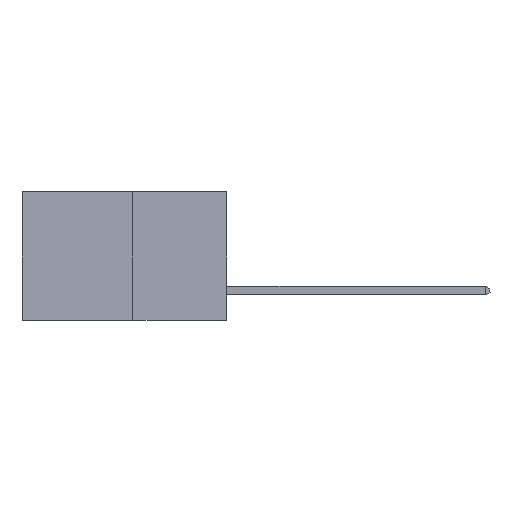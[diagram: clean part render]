
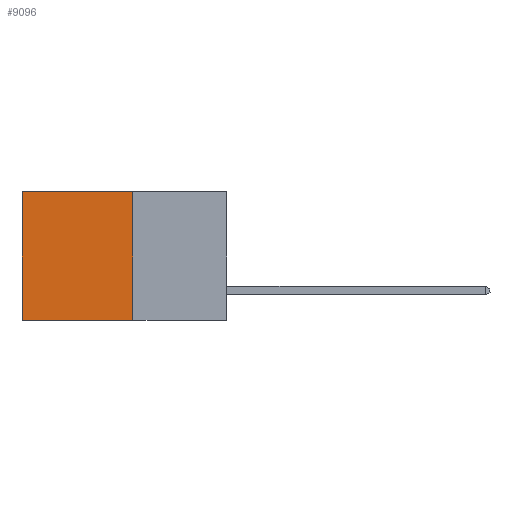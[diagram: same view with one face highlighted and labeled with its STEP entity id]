
A CAD part, left-side view. The second image highlights one B-rep face of the part: STEP entity #9096.
In plain terms, the highlighted planar face has unit normal (-1, 0, 0).
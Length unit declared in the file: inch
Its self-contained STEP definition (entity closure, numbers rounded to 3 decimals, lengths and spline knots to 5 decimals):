
#152 = LINE ( 'NONE', #2036, #10511 ) ;
#272 = VERTEX_POINT ( 'NONE', #1873 ) ;
#310 = VECTOR ( 'NONE', #3339, 39.37008 ) ;
#733 = CARTESIAN_POINT ( 'NONE',  ( 0.277, 0.27, 0. ) ) ;
#773 = ORIENTED_EDGE ( 'NONE', *, *, #8752, .F. ) ;
#1008 = DIRECTION ( 'NONE',  ( 0., 0., -1. ) ) ;
#1807 = DIRECTION ( 'NONE',  ( 1., 0., 0. ) ) ;
#1873 = CARTESIAN_POINT ( 'NONE',  ( 0.277, 0.27, -0.37 ) ) ;
#2036 = CARTESIAN_POINT ( 'NONE',  ( 0.277, 0.27, -0.37 ) ) ;
#2750 = VERTEX_POINT ( 'NONE', #10071 ) ;
#3150 = CARTESIAN_POINT ( 'NONE',  ( 0.277, 0.27, -0.37 ) ) ;
#3339 = DIRECTION ( 'NONE',  ( 0., 1., 0. ) ) ;
#3809 = ORIENTED_EDGE ( 'NONE', *, *, #11280, .T. ) ;
#3997 = CARTESIAN_POINT ( 'NONE',  ( 0.277, 0.59, -0.37 ) ) ;
#4216 = VERTEX_POINT ( 'NONE', #6835 ) ;
#4454 = EDGE_LOOP ( 'NONE', ( #8156, #773, #6133, #3809 ) ) ;
#4616 = VECTOR ( 'NONE', #10073, 39.37008 ) ;
#4999 = DIRECTION ( 'NONE',  ( 0., 0., -1. ) ) ;
#6133 = ORIENTED_EDGE ( 'NONE', *, *, #7423, .F. ) ;
#6651 = VECTOR ( 'NONE', #4999, 39.37008 ) ;
#6835 = CARTESIAN_POINT ( 'NONE',  ( 0.277, 0.59, 0. ) ) ;
#7266 = LINE ( 'NONE', #3150, #4616 ) ;
#7423 = EDGE_CURVE ( 'NONE', #9100, #272, #152, .T. ) ;
#7792 = CARTESIAN_POINT ( 'NONE',  ( 0.277, 0.27, -0.37 ) ) ;
#7883 = FACE_OUTER_BOUND ( 'NONE', #4454, .T. ) ;
#8156 = ORIENTED_EDGE ( 'NONE', *, *, #11171, .T. ) ;
#8288 = CARTESIAN_POINT ( 'NONE',  ( 0.277, 0.27, 0. ) ) ;
#8657 = LINE ( 'NONE', #8288, #310 ) ;
#8746 = DIRECTION ( 'NONE',  ( 0., 0., -1. ) ) ;
#8752 = EDGE_CURVE ( 'NONE', #272, #2750, #7266, .T. ) ;
#9096 = ADVANCED_FACE ( 'NONE', ( #7883 ), #12636, .F. ) ;
#9100 = VERTEX_POINT ( 'NONE', #733 ) ;
#10071 = CARTESIAN_POINT ( 'NONE',  ( 0.277, 0.59, -0.37 ) ) ;
#10073 = DIRECTION ( 'NONE',  ( 0., 1., 0. ) ) ;
#10264 = AXIS2_PLACEMENT_3D ( 'NONE', #7792, #1807, #8746 ) ;
#10511 = VECTOR ( 'NONE', #1008, 39.37008 ) ;
#11171 = EDGE_CURVE ( 'NONE', #4216, #2750, #12170, .T. ) ;
#11280 = EDGE_CURVE ( 'NONE', #9100, #4216, #8657, .T. ) ;
#12170 = LINE ( 'NONE', #3997, #6651 ) ;
#12636 = PLANE ( 'NONE',  #10264 ) ;
